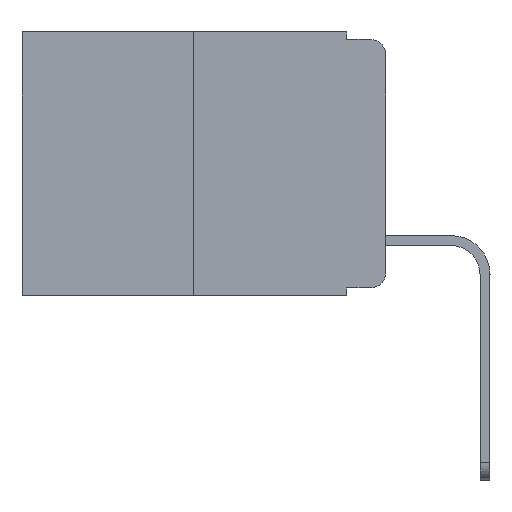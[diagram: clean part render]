
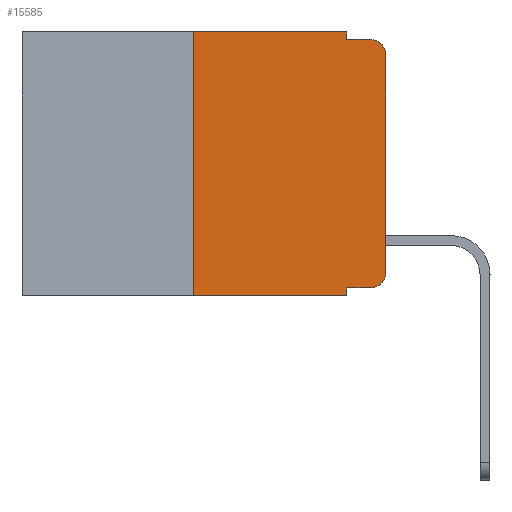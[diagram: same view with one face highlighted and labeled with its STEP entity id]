
A CAD part, left-side view. The second image highlights one B-rep face of the part: STEP entity #15585.
In plain terms, the highlighted planar face has unit normal (-1, 0, 0).
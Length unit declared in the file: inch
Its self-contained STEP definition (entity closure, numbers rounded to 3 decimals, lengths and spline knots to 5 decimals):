
#293 = ORIENTED_EDGE ( 'NONE', *, *, #15971, .T. ) ;
#406 = EDGE_CURVE ( 'NONE', #18593, #20508, #6924, .T. ) ;
#717 = VERTEX_POINT ( 'NONE', #1861 ) ;
#852 = DIRECTION ( 'NONE',  ( 0., -1., 0. ) ) ;
#1606 = CARTESIAN_POINT ( 'NONE',  ( 0., 0.02, -0.03 ) ) ;
#1824 = VERTEX_POINT ( 'NONE', #5207 ) ;
#1835 = CARTESIAN_POINT ( 'NONE',  ( 0., 0.051, 0. ) ) ;
#1861 = CARTESIAN_POINT ( 'NONE',  ( 0., 0.051, -0.333 ) ) ;
#2199 = VERTEX_POINT ( 'NONE', #20515 ) ;
#2227 = DIRECTION ( 'NONE',  ( 0., 0., -1. ) ) ;
#2286 = AXIS2_PLACEMENT_3D ( 'NONE', #24325, #10365, #12456 ) ;
#2320 = LINE ( 'NONE', #10834, #6081 ) ;
#2489 = ORIENTED_EDGE ( 'NONE', *, *, #20538, .T. ) ;
#3798 = DIRECTION ( 'NONE',  ( 0., 0., -1. ) ) ;
#3804 = ORIENTED_EDGE ( 'NONE', *, *, #15581, .F. ) ;
#4152 = CARTESIAN_POINT ( 'NONE',  ( 0., 0.051, 0. ) ) ;
#4509 = CARTESIAN_POINT ( 'NONE',  ( 0., 0.051, -0.343 ) ) ;
#4692 = VERTEX_POINT ( 'NONE', #6596 ) ;
#4859 = CARTESIAN_POINT ( 'NONE',  ( 0., 0.051, -0.01 ) ) ;
#4876 = CARTESIAN_POINT ( 'NONE',  ( 0., 0.25, 0. ) ) ;
#4980 = EDGE_CURVE ( 'NONE', #717, #14300, #2320, .T. ) ;
#5207 = CARTESIAN_POINT ( 'NONE',  ( 0., 0.25, -0.343 ) ) ;
#5958 = CARTESIAN_POINT ( 'NONE',  ( 0., 0.473, 0. ) ) ;
#6081 = VECTOR ( 'NONE', #8967, 39.37008 ) ;
#6226 = DIRECTION ( 'NONE',  ( 0., -1., 0. ) ) ;
#6596 = CARTESIAN_POINT ( 'NONE',  ( 0., 0.02, -0.01 ) ) ;
#6924 = LINE ( 'NONE', #11838, #8508 ) ;
#7370 = VECTOR ( 'NONE', #8082, 39.37008 ) ;
#8082 = DIRECTION ( 'NONE',  ( 0., 0., -1. ) ) ;
#8307 = VECTOR ( 'NONE', #852, 39.37008 ) ;
#8414 = ORIENTED_EDGE ( 'NONE', *, *, #16888, .T. ) ;
#8508 = VECTOR ( 'NONE', #6226, 39.37008 ) ;
#8541 = VERTEX_POINT ( 'NONE', #4509 ) ;
#8589 = VERTEX_POINT ( 'NONE', #4859 ) ;
#8617 = LINE ( 'NONE', #18972, #8307 ) ;
#8967 = DIRECTION ( 'NONE',  ( 0., -1., 0. ) ) ;
#9804 = DIRECTION ( 'NONE',  ( -1., 0., 0. ) ) ;
#10365 = DIRECTION ( 'NONE',  ( -1., 0., 0. ) ) ;
#10834 = CARTESIAN_POINT ( 'NONE',  ( 0., 0.051, -0.333 ) ) ;
#11838 = CARTESIAN_POINT ( 'NONE',  ( 0., 0.473, 0. ) ) ;
#11938 = DIRECTION ( 'NONE',  ( 1., 0., 0. ) ) ;
#12020 = CARTESIAN_POINT ( 'NONE',  ( 0., 0.051, -0.01 ) ) ;
#12332 = EDGE_CURVE ( 'NONE', #26070, #2199, #12766, .T. ) ;
#12456 = DIRECTION ( 'NONE',  ( 0., 0., -1. ) ) ;
#12766 = LINE ( 'NONE', #23334, #17237 ) ;
#13492 = ORIENTED_EDGE ( 'NONE', *, *, #12332, .T. ) ;
#14032 = AXIS2_PLACEMENT_3D ( 'NONE', #1606, #9804, #3798 ) ;
#14230 = LINE ( 'NONE', #4152, #21573 ) ;
#14248 = DIRECTION ( 'NONE',  ( 0., 0., -1. ) ) ;
#14300 = VERTEX_POINT ( 'NONE', #24220 ) ;
#14303 = VECTOR ( 'NONE', #22285, 39.37008 ) ;
#15081 = ORIENTED_EDGE ( 'NONE', *, *, #4980, .T. ) ;
#15581 = EDGE_CURVE ( 'NONE', #20508, #8589, #24863, .T. ) ;
#15585 = ADVANCED_FACE ( 'NONE', ( #19402 ), #20399, .F. ) ;
#15688 = ORIENTED_EDGE ( 'NONE', *, *, #406, .F. ) ;
#15855 = EDGE_CURVE ( 'NONE', #8589, #4692, #17794, .T. ) ;
#15934 = EDGE_CURVE ( 'NONE', #1824, #18593, #26112, .T. ) ;
#15971 = EDGE_CURVE ( 'NONE', #1824, #8541, #8617, .T. ) ;
#16113 = CARTESIAN_POINT ( 'NONE',  ( 0., 0.25, 0. ) ) ;
#16421 = EDGE_LOOP ( 'NONE', ( #13492, #8414, #17152, #3804, #15688, #19246, #293, #25420, #15081, #2489 ) ) ;
#16888 = EDGE_CURVE ( 'NONE', #2199, #4692, #19974, .T. ) ;
#17007 = EDGE_CURVE ( 'NONE', #717, #8541, #14230, .T. ) ;
#17152 = ORIENTED_EDGE ( 'NONE', *, *, #15855, .F. ) ;
#17237 = VECTOR ( 'NONE', #23962, 39.37008 ) ;
#17794 = LINE ( 'NONE', #12020, #14303 ) ;
#18593 = VERTEX_POINT ( 'NONE', #4876 ) ;
#18972 = CARTESIAN_POINT ( 'NONE',  ( 0., 0.473, -0.343 ) ) ;
#19246 = ORIENTED_EDGE ( 'NONE', *, *, #15934, .F. ) ;
#19402 = FACE_OUTER_BOUND ( 'NONE', #16421, .T. ) ;
#19974 = CIRCLE ( 'NONE', #14032, 0.02 ) ;
#20399 = PLANE ( 'NONE',  #26164 ) ;
#20508 = VERTEX_POINT ( 'NONE', #24062 ) ;
#20515 = CARTESIAN_POINT ( 'NONE',  ( 0., 0., -0.03 ) ) ;
#20538 = EDGE_CURVE ( 'NONE', #14300, #26070, #25126, .T. ) ;
#21573 = VECTOR ( 'NONE', #2227, 39.37008 ) ;
#21586 = CARTESIAN_POINT ( 'NONE',  ( 0., 0., -0.313 ) ) ;
#21963 = VECTOR ( 'NONE', #24245, 39.37008 ) ;
#22285 = DIRECTION ( 'NONE',  ( 0., -1., 0. ) ) ;
#23334 = CARTESIAN_POINT ( 'NONE',  ( 0., 0., 0. ) ) ;
#23962 = DIRECTION ( 'NONE',  ( 0., 0., 1. ) ) ;
#24062 = CARTESIAN_POINT ( 'NONE',  ( 0., 0.051, 0. ) ) ;
#24220 = CARTESIAN_POINT ( 'NONE',  ( 0., 0.02, -0.333 ) ) ;
#24245 = DIRECTION ( 'NONE',  ( 0., 0., 1. ) ) ;
#24325 = CARTESIAN_POINT ( 'NONE',  ( 0., 0.02, -0.313 ) ) ;
#24863 = LINE ( 'NONE', #1835, #7370 ) ;
#25126 = CIRCLE ( 'NONE', #2286, 0.02 ) ;
#25420 = ORIENTED_EDGE ( 'NONE', *, *, #17007, .F. ) ;
#26070 = VERTEX_POINT ( 'NONE', #21586 ) ;
#26112 = LINE ( 'NONE', #16113, #21963 ) ;
#26164 = AXIS2_PLACEMENT_3D ( 'NONE', #5958, #11938, #14248 ) ;
